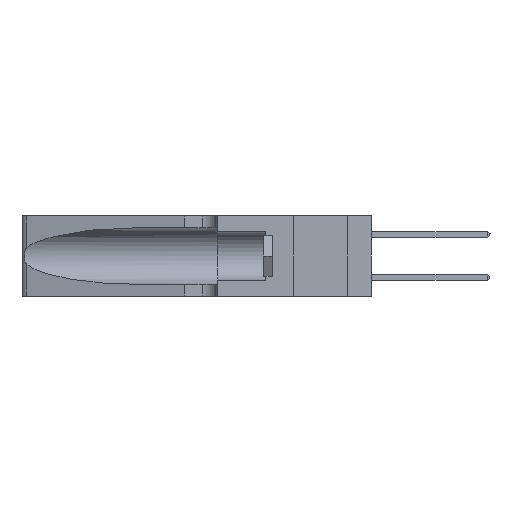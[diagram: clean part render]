
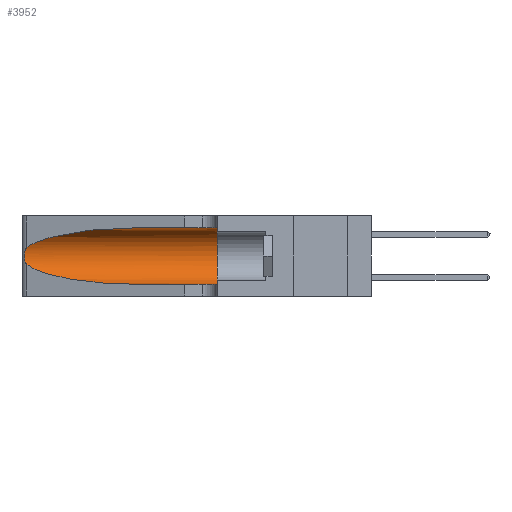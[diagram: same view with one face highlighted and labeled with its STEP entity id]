
A CAD part, left-side view. The second image highlights one B-rep face of the part: STEP entity #3952.
In plain terms, the highlighted cylindrical face has radius 3.308 mm (diameter 6.617 mm), a partial arc.
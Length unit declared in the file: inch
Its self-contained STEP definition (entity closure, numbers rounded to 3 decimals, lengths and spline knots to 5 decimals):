
#363 = CARTESIAN_POINT ( 'NONE',  ( 0.1305, 0.72297, 0.31525 ) ) ;
#364 = CARTESIAN_POINT ( 'NONE',  ( 0.18966, 0.96281, 0.05475 ) ) ;
#978 = CARTESIAN_POINT ( 'NONE',  ( 0.1305, 1.61858, 0.05475 ) ) ;
#1216 = CARTESIAN_POINT ( 'NONE',  ( 0.25487, 1.22718, 0.22369 ) ) ;
#1417 = ORIENTED_EDGE ( 'NONE', *, *, #22131, .T. ) ;
#1734 = CARTESIAN_POINT ( 'NONE',  ( 0.25639, 1.23184, 0.21858 ) ) ;
#1788 = AXIS2_PLACEMENT_3D ( 'NONE', #18062, #6249, #24085 ) ;
#3026 = CARTESIAN_POINT ( 'NONE',  ( 0.1305, 0.72297, 0.31525 ) ) ;
#3470 = CARTESIAN_POINT ( 'NONE',  ( 0.1305, 0.35, 0.05475 ) ) ;
#3778 = VERTEX_POINT ( 'NONE', #3470 ) ;
#3926 = DIRECTION ( 'NONE',  ( 0., -1., 0. ) ) ;
#3952 = ADVANCED_FACE ( 'NONE', ( #21179 ), #21470, .F. ) ;
#3994 =( BOUNDED_CURVE ( )  B_SPLINE_CURVE ( 3, ( #24160, #12570, #364, #14555 ),
 .UNSPECIFIED., .F., .F. ) 
 B_SPLINE_CURVE_WITH_KNOTS ( ( 4, 4 ),
 ( 3.44316, 4.71239 ),
 .UNSPECIFIED. ) 
 CURVE ( )  GEOMETRIC_REPRESENTATION_ITEM ( )  RATIONAL_B_SPLINE_CURVE ( ( 1., 0.87, 0.87, 1. ) ) 
 REPRESENTATION_ITEM ( '' )  );
#4200 = ORIENTED_EDGE ( 'NONE', *, *, #17065, .F. ) ;
#4695 = LINE ( 'NONE', #13794, #16451 ) ;
#5036 = CARTESIAN_POINT ( 'NONE',  ( 0.18966, 0.96281, 0.31525 ) ) ;
#5176 = ORIENTED_EDGE ( 'NONE', *, *, #7591, .T. ) ;
#5657 = CARTESIAN_POINT ( 'NONE',  ( 0.1305, 0.35, 0.31525 ) ) ;
#5949 = CARTESIAN_POINT ( 'NONE',  ( 0.1305, 1.61858, 0.185 ) ) ;
#6180 = CARTESIAN_POINT ( 'NONE',  ( 0.25487, 1.22718, 0.14631 ) ) ;
#6249 = DIRECTION ( 'NONE',  ( 0., 1., 0. ) ) ;
#6391 = CARTESIAN_POINT ( 'NONE',  ( 0.26017, 1.23833, 0.17102 ) ) ;
#6487 = CARTESIAN_POINT ( 'NONE',  ( 0.25487, 1.22718, 0.14631 ) ) ;
#7172 = DIRECTION ( 'NONE',  ( 0., 0., -1. ) ) ;
#7480 = VERTEX_POINT ( 'NONE', #16986 ) ;
#7591 = EDGE_CURVE ( 'NONE', #17298, #20672, #13200, .T. ) ;
#8231 = CARTESIAN_POINT ( 'NONE',  ( 0.25856, 1.23593, 0.16098 ) ) ;
#8612 = B_SPLINE_CURVE_WITH_KNOTS ( 'NONE', 3,
 ( #1216, #15239, #1734, #15730, #17694, #16323, #15992, #18198, #6391, #8231, #16073, #18283, #21988, #6487 ),
 .UNSPECIFIED., .F., .F.,
 ( 4, 2, 2, 2, 2, 2, 4 ),
 ( 0., 0.00027, 0.00053, 0.00107, 0.0016, 0.00187, 0.00214 ),
 .UNSPECIFIED. ) ;
#9799 = EDGE_CURVE ( 'NONE', #7480, #3778, #21180, .T. ) ;
#11357 = VECTOR ( 'NONE', #16867, 39.37008 ) ;
#12564 = ORIENTED_EDGE ( 'NONE', *, *, #18202, .T. ) ;
#12570 = CARTESIAN_POINT ( 'NONE',  ( 0.2373, 1.15595, 0.08982 ) ) ;
#13200 =( BOUNDED_CURVE ( )  B_SPLINE_CURVE ( 3, ( #363, #5036, #21657, #17865 ),
 .UNSPECIFIED., .F., .T. ) 
 B_SPLINE_CURVE_WITH_KNOTS ( ( 4, 4 ),
 ( 1.5708, 2.84003 ),
 .UNSPECIFIED. ) 
 CURVE ( )  GEOMETRIC_REPRESENTATION_ITEM ( )  RATIONAL_B_SPLINE_CURVE ( ( 1., 0.87, 0.87, 1. ) ) 
 REPRESENTATION_ITEM ( '' )  );
#13794 = CARTESIAN_POINT ( 'NONE',  ( 0.1305, 1.61858, 0.31525 ) ) ;
#14555 = CARTESIAN_POINT ( 'NONE',  ( 0.1305, 0.72297, 0.05475 ) ) ;
#15239 = CARTESIAN_POINT ( 'NONE',  ( 0.25555, 1.22994, 0.2215 ) ) ;
#15730 = CARTESIAN_POINT ( 'NONE',  ( 0.25787, 1.23484, 0.2124 ) ) ;
#15992 = CARTESIAN_POINT ( 'NONE',  ( 0.26075, 1.23896, 0.19203 ) ) ;
#16073 = CARTESIAN_POINT ( 'NONE',  ( 0.25789, 1.23486, 0.15765 ) ) ;
#16323 = CARTESIAN_POINT ( 'NONE',  ( 0.26018, 1.23835, 0.19895 ) ) ;
#16451 = VECTOR ( 'NONE', #3926, 39.37008 ) ;
#16534 = AXIS2_PLACEMENT_3D ( 'NONE', #5949, #23958, #7172 ) ;
#16867 = DIRECTION ( 'NONE',  ( 0., -1., 0. ) ) ;
#16986 = CARTESIAN_POINT ( 'NONE',  ( 0.1305, 0.72297, 0.05475 ) ) ;
#17052 = CIRCLE ( 'NONE', #1788, 0.13025 ) ;
#17065 = EDGE_CURVE ( 'NONE', #21775, #3778, #17052, .T. ) ;
#17298 = VERTEX_POINT ( 'NONE', #3026 ) ;
#17694 = CARTESIAN_POINT ( 'NONE',  ( 0.25854, 1.2359, 0.20912 ) ) ;
#17865 = CARTESIAN_POINT ( 'NONE',  ( 0.25487, 1.22718, 0.22369 ) ) ;
#18062 = CARTESIAN_POINT ( 'NONE',  ( 0.1305, 0.35, 0.185 ) ) ;
#18198 = CARTESIAN_POINT ( 'NONE',  ( 0.26075, 1.23896, 0.178 ) ) ;
#18202 = EDGE_CURVE ( 'NONE', #20672, #25166, #8612, .T. ) ;
#18283 = CARTESIAN_POINT ( 'NONE',  ( 0.25639, 1.23186, 0.15144 ) ) ;
#18926 = EDGE_CURVE ( 'NONE', #17298, #21775, #4695, .T. ) ;
#19027 = ORIENTED_EDGE ( 'NONE', *, *, #18926, .F. ) ;
#19786 = CARTESIAN_POINT ( 'NONE',  ( 0.25487, 1.22718, 0.22369 ) ) ;
#20672 = VERTEX_POINT ( 'NONE', #19786 ) ;
#21179 = FACE_OUTER_BOUND ( 'NONE', #22230, .T. ) ;
#21180 = LINE ( 'NONE', #978, #11357 ) ;
#21470 = CYLINDRICAL_SURFACE ( 'NONE', #16534, 0.13025 ) ;
#21657 = CARTESIAN_POINT ( 'NONE',  ( 0.2373, 1.15595, 0.28018 ) ) ;
#21775 = VERTEX_POINT ( 'NONE', #5657 ) ;
#21988 = CARTESIAN_POINT ( 'NONE',  ( 0.25555, 1.22993, 0.14849 ) ) ;
#22131 = EDGE_CURVE ( 'NONE', #25166, #7480, #3994, .T. ) ;
#22230 = EDGE_LOOP ( 'NONE', ( #5176, #12564, #1417, #22742, #4200, #19027 ) ) ;
#22742 = ORIENTED_EDGE ( 'NONE', *, *, #9799, .T. ) ;
#23958 = DIRECTION ( 'NONE',  ( 0., -1., 0. ) ) ;
#24085 = DIRECTION ( 'NONE',  ( 0., 0., 1. ) ) ;
#24160 = CARTESIAN_POINT ( 'NONE',  ( 0.25487, 1.22718, 0.14631 ) ) ;
#25166 = VERTEX_POINT ( 'NONE', #6180 ) ;
